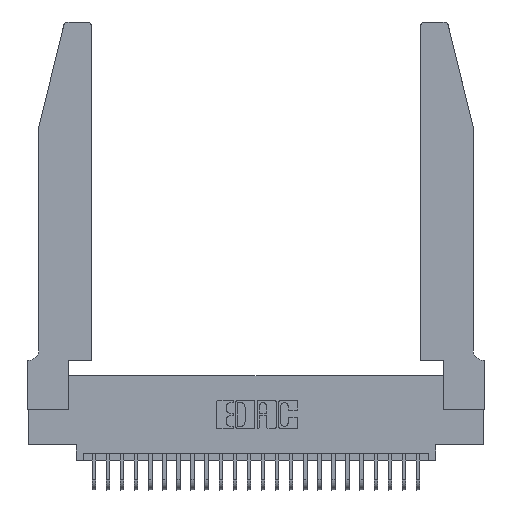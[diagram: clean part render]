
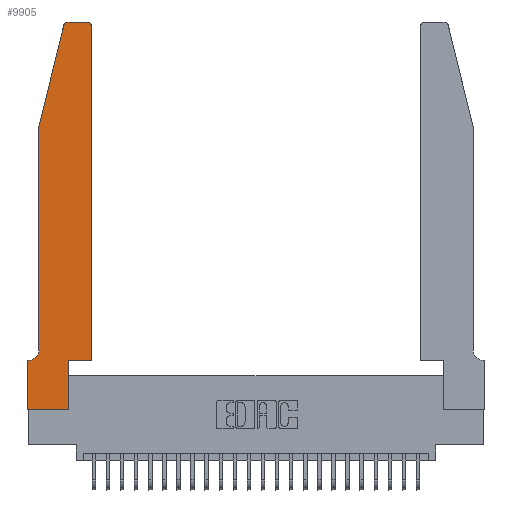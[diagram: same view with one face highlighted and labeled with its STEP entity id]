
A CAD part, top view. The second image highlights one B-rep face of the part: STEP entity #9905.
In plain terms, the highlighted planar face has unit normal (0, 0, 1).
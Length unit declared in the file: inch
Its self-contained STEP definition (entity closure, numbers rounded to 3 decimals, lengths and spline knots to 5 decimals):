
#1208 = VECTOR ( 'NONE', #16602, 39.37008 ) ;
#1246 = CARTESIAN_POINT ( 'NONE',  ( 0.4205, 2.75, 0.37 ) ) ;
#1763 = EDGE_CURVE ( 'NONE', #12259, #16869, #4402, .T. ) ;
#2085 = DIRECTION ( 'NONE',  ( 1., 0., 0. ) ) ;
#2253 = DIRECTION ( 'NONE',  ( 0., 0., 1. ) ) ;
#2311 = ORIENTED_EDGE ( 'NONE', *, *, #19000, .T. ) ;
#2678 = CARTESIAN_POINT ( 'NONE',  ( 0., 0., 0.37 ) ) ;
#2698 = ORIENTED_EDGE ( 'NONE', *, *, #19170, .T. ) ;
#2839 = LINE ( 'NONE', #27367, #13638 ) ;
#2912 = CARTESIAN_POINT ( 'NONE',  ( 0., 0., 0.37 ) ) ;
#3132 = CARTESIAN_POINT ( 'NONE',  ( 0., 0.35, 0.37 ) ) ;
#3190 = ORIENTED_EDGE ( 'NONE', *, *, #19146, .T. ) ;
#3295 = ORIENTED_EDGE ( 'NONE', *, *, #9433, .T. ) ;
#3589 = CARTESIAN_POINT ( 'NONE',  ( 0.0055, 0.35, 0.37 ) ) ;
#3748 = CARTESIAN_POINT ( 'NONE',  ( 0.25487, 2.72718, 0.37 ) ) ;
#3943 = VECTOR ( 'NONE', #17985, 39.37008 ) ;
#4086 = CARTESIAN_POINT ( 'NONE',  ( 0.4505, 0.35, 0.37 ) ) ;
#4244 = CIRCLE ( 'NONE', #19566, 0.03 ) ;
#4285 = VERTEX_POINT ( 'NONE', #3589 ) ;
#4373 = VERTEX_POINT ( 'NONE', #8188 ) ;
#4402 = CIRCLE ( 'NONE', #15142, 0.03 ) ;
#4533 = DIRECTION ( 'NONE',  ( 0., 0., -1. ) ) ;
#4937 = EDGE_CURVE ( 'NONE', #11869, #20662, #14048, .T. ) ;
#5020 = CARTESIAN_POINT ( 'NONE',  ( 0.0755, 0.35, 0.37 ) ) ;
#5113 = DIRECTION ( 'NONE',  ( 0., -1., 0. ) ) ;
#5165 = PLANE ( 'NONE',  #26538 ) ;
#5261 = DIRECTION ( 'NONE',  ( 1., 0., 0. ) ) ;
#5280 = VECTOR ( 'NONE', #17523, 39.37008 ) ;
#5640 = VECTOR ( 'NONE', #8977, 39.37008 ) ;
#5827 = CIRCLE ( 'NONE', #23581, 0.07 ) ;
#5970 = LINE ( 'NONE', #8810, #5280 ) ;
#6205 = ORIENTED_EDGE ( 'NONE', *, *, #12782, .T. ) ;
#6320 = ORIENTED_EDGE ( 'NONE', *, *, #22997, .T. ) ;
#7056 = EDGE_CURVE ( 'NONE', #15257, #9518, #23491, .T. ) ;
#7073 = EDGE_CURVE ( 'NONE', #24713, #14280, #22162, .T. ) ;
#7820 = VERTEX_POINT ( 'NONE', #14006 ) ;
#8188 = CARTESIAN_POINT ( 'NONE',  ( 0.284, 2.75, 0.37 ) ) ;
#8324 = LINE ( 'NONE', #5020, #3943 ) ;
#8674 = ORIENTED_EDGE ( 'NONE', *, *, #7056, .T. ) ;
#8810 = CARTESIAN_POINT ( 'NONE',  ( 0.2605, 2.75, 0.37 ) ) ;
#8977 = DIRECTION ( 'NONE',  ( 1., 0., 0. ) ) ;
#9433 = EDGE_CURVE ( 'NONE', #14280, #15257, #2839, .T. ) ;
#9445 = CARTESIAN_POINT ( 'NONE',  ( 0.4505, 0.35, 0.37 ) ) ;
#9518 = VERTEX_POINT ( 'NONE', #4086 ) ;
#9905 = ADVANCED_FACE ( 'NONE', ( #25650 ), #5165, .T. ) ;
#10734 = ORIENTED_EDGE ( 'NONE', *, *, #16100, .T. ) ;
#11061 = ORIENTED_EDGE ( 'NONE', *, *, #7073, .T. ) ;
#11536 = VECTOR ( 'NONE', #17765, 39.37008 ) ;
#11869 = VERTEX_POINT ( 'NONE', #3748 ) ;
#12259 = VERTEX_POINT ( 'NONE', #22343 ) ;
#12398 = DIRECTION ( 'NONE',  ( 0., 1., 0. ) ) ;
#12782 = EDGE_CURVE ( 'NONE', #7820, #4285, #5827, .T. ) ;
#12934 = CARTESIAN_POINT ( 'NONE',  ( 0., 0.35, 0.37 ) ) ;
#13283 = CARTESIAN_POINT ( 'NONE',  ( 0., 0., 0.37 ) ) ;
#13373 = DIRECTION ( 'NONE',  ( 1., 0., 0. ) ) ;
#13638 = VECTOR ( 'NONE', #12398, 39.37008 ) ;
#14006 = CARTESIAN_POINT ( 'NONE',  ( 0.0755, 0.42, 0.37 ) ) ;
#14048 = LINE ( 'NONE', #18742, #1208 ) ;
#14108 = LINE ( 'NONE', #18072, #24788 ) ;
#14280 = VERTEX_POINT ( 'NONE', #17202 ) ;
#14292 = VERTEX_POINT ( 'NONE', #12934 ) ;
#15030 = DIRECTION ( 'NONE',  ( 0., 0., 1. ) ) ;
#15142 = AXIS2_PLACEMENT_3D ( 'NONE', #15200, #2253, #17349 ) ;
#15200 = CARTESIAN_POINT ( 'NONE',  ( 0.4205, 2.72, 0.37 ) ) ;
#15257 = VERTEX_POINT ( 'NONE', #20800 ) ;
#16100 = EDGE_CURVE ( 'NONE', #9518, #12259, #18505, .T. ) ;
#16505 = VECTOR ( 'NONE', #13373, 39.37008 ) ;
#16602 = DIRECTION ( 'NONE',  ( -0.239, -0.971, 0. ) ) ;
#16869 = VERTEX_POINT ( 'NONE', #1246 ) ;
#17063 = CARTESIAN_POINT ( 'NONE',  ( 0.0755, 2., 0.37 ) ) ;
#17139 = EDGE_CURVE ( 'NONE', #4373, #11869, #4244, .T. ) ;
#17202 = CARTESIAN_POINT ( 'NONE',  ( 0.2865, 0., 0.37 ) ) ;
#17349 = DIRECTION ( 'NONE',  ( 1., 0., 0. ) ) ;
#17486 = CARTESIAN_POINT ( 'NONE',  ( 0.0055, 0.42, 0.37 ) ) ;
#17523 = DIRECTION ( 'NONE',  ( -1., 0., 0. ) ) ;
#17765 = DIRECTION ( 'NONE',  ( 0., -1., 0. ) ) ;
#17826 = VECTOR ( 'NONE', #26609, 39.37008 ) ;
#17908 = EDGE_LOOP ( 'NONE', ( #2311, #20874, #25863, #2698, #6205, #3190, #6320, #11061, #3295, #8674, #10734, #26838 ) ) ;
#17985 = DIRECTION ( 'NONE',  ( -1., 0., 0. ) ) ;
#18072 = CARTESIAN_POINT ( 'NONE',  ( 0.0755, 2., 0.37 ) ) ;
#18233 = DIRECTION ( 'NONE',  ( 0., 0., 1. ) ) ;
#18505 = LINE ( 'NONE', #9445, #17826 ) ;
#18742 = CARTESIAN_POINT ( 'NONE',  ( 0.0755, 2., 0.37 ) ) ;
#19000 = EDGE_CURVE ( 'NONE', #16869, #4373, #5970, .T. ) ;
#19146 = EDGE_CURVE ( 'NONE', #4285, #14292, #8324, .T. ) ;
#19170 = EDGE_CURVE ( 'NONE', #20662, #7820, #14108, .T. ) ;
#19566 = AXIS2_PLACEMENT_3D ( 'NONE', #27781, #15030, #2085 ) ;
#19649 = DIRECTION ( 'NONE',  ( -1., 0., 0. ) ) ;
#20662 = VERTEX_POINT ( 'NONE', #17063 ) ;
#20800 = CARTESIAN_POINT ( 'NONE',  ( 0.2865, 0.35, 0.37 ) ) ;
#20874 = ORIENTED_EDGE ( 'NONE', *, *, #17139, .T. ) ;
#21898 = CARTESIAN_POINT ( 'NONE',  ( 0.4505, 0.35, 0.37 ) ) ;
#22162 = LINE ( 'NONE', #13283, #16505 ) ;
#22343 = CARTESIAN_POINT ( 'NONE',  ( 0.4505, 2.72, 0.37 ) ) ;
#22997 = EDGE_CURVE ( 'NONE', #14292, #24713, #23626, .T. ) ;
#23491 = LINE ( 'NONE', #21898, #5640 ) ;
#23581 = AXIS2_PLACEMENT_3D ( 'NONE', #17486, #4533, #19649 ) ;
#23626 = LINE ( 'NONE', #2678, #11536 ) ;
#24713 = VERTEX_POINT ( 'NONE', #2912 ) ;
#24788 = VECTOR ( 'NONE', #5113, 39.37008 ) ;
#25650 = FACE_OUTER_BOUND ( 'NONE', #17908, .T. ) ;
#25863 = ORIENTED_EDGE ( 'NONE', *, *, #4937, .T. ) ;
#26538 = AXIS2_PLACEMENT_3D ( 'NONE', #3132, #18233, #5261 ) ;
#26609 = DIRECTION ( 'NONE',  ( 0., 1., 0. ) ) ;
#26838 = ORIENTED_EDGE ( 'NONE', *, *, #1763, .T. ) ;
#27367 = CARTESIAN_POINT ( 'NONE',  ( 0.2865, 0.35, 0.37 ) ) ;
#27781 = CARTESIAN_POINT ( 'NONE',  ( 0.284, 2.72, 0.37 ) ) ;
